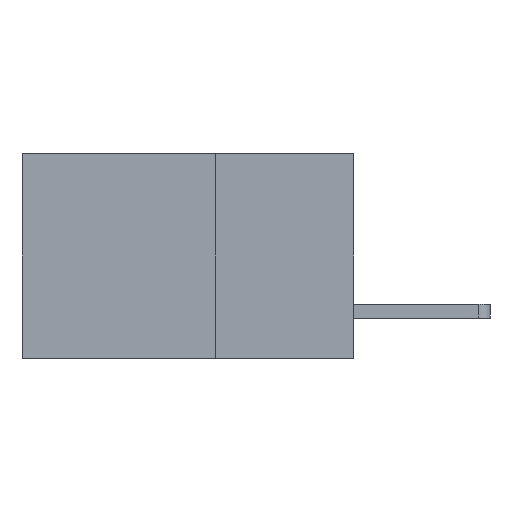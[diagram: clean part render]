
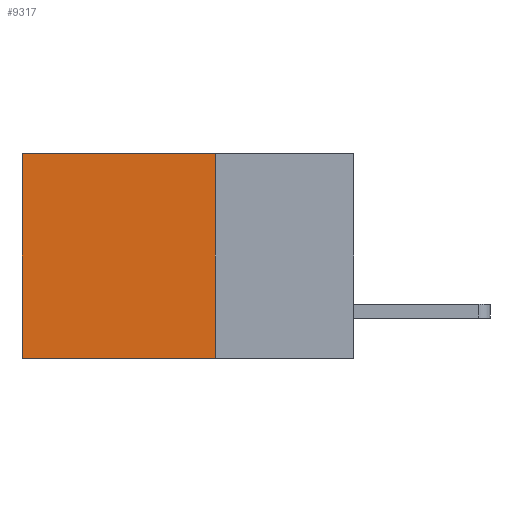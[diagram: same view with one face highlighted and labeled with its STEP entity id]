
A CAD part, left-side view. The second image highlights one B-rep face of the part: STEP entity #9317.
In plain terms, the highlighted planar face has unit normal (-1, 0, 0).
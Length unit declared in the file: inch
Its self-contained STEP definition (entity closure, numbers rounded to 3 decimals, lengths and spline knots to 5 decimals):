
#35 = VERTEX_POINT ( 'NONE', #5443 ) ;
#164 = DIRECTION ( 'NONE',  ( 1., 0., 0. ) ) ;
#453 = VECTOR ( 'NONE', #6919, 39.37008 ) ;
#685 = ORIENTED_EDGE ( 'NONE', *, *, #2379, .T. ) ;
#698 = VECTOR ( 'NONE', #8700, 39.37008 ) ;
#719 = ORIENTED_EDGE ( 'NONE', *, *, #8580, .T. ) ;
#965 = CARTESIAN_POINT ( 'NONE',  ( 0.2875, 0.6, 0. ) ) ;
#2379 = EDGE_CURVE ( 'NONE', #8556, #35, #6035, .T. ) ;
#2906 = ORIENTED_EDGE ( 'NONE', *, *, #4277, .F. ) ;
#3273 = CARTESIAN_POINT ( 'NONE',  ( 0.2875, 0.25, -0.37 ) ) ;
#3550 = VECTOR ( 'NONE', #7618, 39.37008 ) ;
#3634 = CARTESIAN_POINT ( 'NONE',  ( 0.2875, 0.25, 0. ) ) ;
#4070 = AXIS2_PLACEMENT_3D ( 'NONE', #6037, #164, #6069 ) ;
#4277 = EDGE_CURVE ( 'NONE', #5905, #35, #5209, .T. ) ;
#4506 = CARTESIAN_POINT ( 'NONE',  ( 0.2875, 0.6, 0. ) ) ;
#4700 = DIRECTION ( 'NONE',  ( 0., 0., -1. ) ) ;
#5209 = LINE ( 'NONE', #8660, #698 ) ;
#5443 = CARTESIAN_POINT ( 'NONE',  ( 0.2875, 0.6, -0.37 ) ) ;
#5877 = CARTESIAN_POINT ( 'NONE',  ( 0.2875, 0.25, 0. ) ) ;
#5905 = VERTEX_POINT ( 'NONE', #3273 ) ;
#6035 = LINE ( 'NONE', #965, #3550 ) ;
#6037 = CARTESIAN_POINT ( 'NONE',  ( 0.2875, 0.25, 0. ) ) ;
#6069 = DIRECTION ( 'NONE',  ( 0., 0., -1. ) ) ;
#6919 = DIRECTION ( 'NONE',  ( 0., 1., 0. ) ) ;
#7073 = LINE ( 'NONE', #3634, #453 ) ;
#7618 = DIRECTION ( 'NONE',  ( 0., 0., -1. ) ) ;
#7643 = ORIENTED_EDGE ( 'NONE', *, *, #9471, .F. ) ;
#8556 = VERTEX_POINT ( 'NONE', #4506 ) ;
#8580 = EDGE_CURVE ( 'NONE', #10392, #8556, #7073, .T. ) ;
#8634 = CARTESIAN_POINT ( 'NONE',  ( 0.2875, 0.25, 0. ) ) ;
#8660 = CARTESIAN_POINT ( 'NONE',  ( 0.2875, 0.25, -0.37 ) ) ;
#8700 = DIRECTION ( 'NONE',  ( 0., 1., 0. ) ) ;
#8789 = EDGE_LOOP ( 'NONE', ( #685, #2906, #7643, #719 ) ) ;
#9158 = PLANE ( 'NONE',  #4070 ) ;
#9317 = ADVANCED_FACE ( 'NONE', ( #10345 ), #9158, .F. ) ;
#9471 = EDGE_CURVE ( 'NONE', #10392, #5905, #10204, .T. ) ;
#9968 = VECTOR ( 'NONE', #4700, 39.37008 ) ;
#10204 = LINE ( 'NONE', #8634, #9968 ) ;
#10345 = FACE_OUTER_BOUND ( 'NONE', #8789, .T. ) ;
#10392 = VERTEX_POINT ( 'NONE', #5877 ) ;
